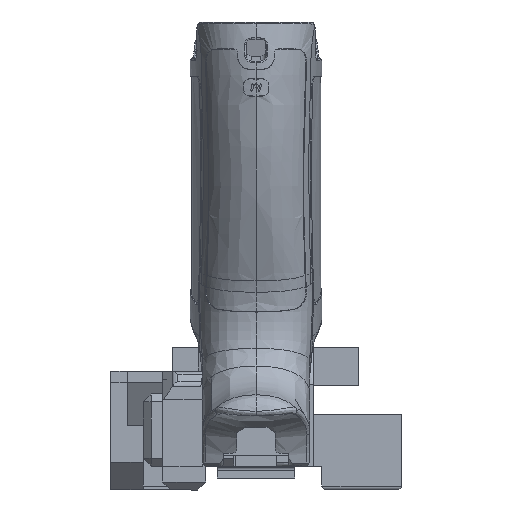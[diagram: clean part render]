
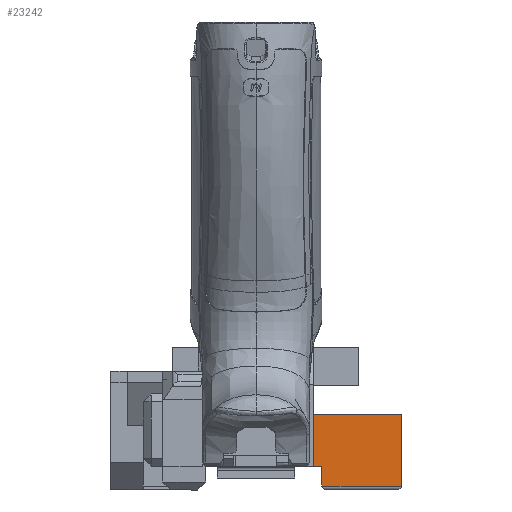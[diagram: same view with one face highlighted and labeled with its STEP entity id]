
A CAD part, left-side view. The second image highlights one B-rep face of the part: STEP entity #23242.
In plain terms, the highlighted planar face has unit normal (-1, 0, 0).
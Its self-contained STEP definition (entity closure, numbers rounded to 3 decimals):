
#552=CIRCLE('',#24701,3.);
#1266=PLANE('',#24794);
#2491=FACE_OUTER_BOUND('',#3825,.T.);
#3825=EDGE_LOOP('',(#18093,#18094,#18095,#18096,#18097,#18098,#18099));
#6152=LINE('',#62624,#8040);
#6186=LINE('',#62721,#8074);
#6187=LINE('',#62723,#8075);
#6188=LINE('',#62725,#8076);
#6189=LINE('',#62726,#8077);
#6190=LINE('',#62727,#8078);
#8040=VECTOR('',#27793,10.);
#8074=VECTOR('',#27853,10.);
#8075=VECTOR('',#27854,10.);
#8076=VECTOR('',#27855,10.);
#8077=VECTOR('',#27856,10.);
#8078=VECTOR('',#27857,10.);
#10216=VERTEX_POINT('',#59979);
#10222=VERTEX_POINT('',#60356);
#10321=VERTEX_POINT('',#62622);
#10356=VERTEX_POINT('',#62719);
#10357=VERTEX_POINT('',#62720);
#10358=VERTEX_POINT('',#62722);
#10359=VERTEX_POINT('',#62724);
#12967=EDGE_CURVE('',#10216,#10222,#552,.T.);
#13136=EDGE_CURVE('',#10216,#10321,#6152,.T.);
#13178=EDGE_CURVE('',#10356,#10357,#6186,.T.);
#13179=EDGE_CURVE('',#10358,#10356,#6187,.T.);
#13180=EDGE_CURVE('',#10359,#10358,#6188,.T.);
#13181=EDGE_CURVE('',#10222,#10359,#6189,.T.);
#13182=EDGE_CURVE('',#10321,#10357,#6190,.T.);
#18093=ORIENTED_EDGE('',*,*,#13178,.F.);
#18094=ORIENTED_EDGE('',*,*,#13179,.F.);
#18095=ORIENTED_EDGE('',*,*,#13180,.F.);
#18096=ORIENTED_EDGE('',*,*,#13181,.F.);
#18097=ORIENTED_EDGE('',*,*,#12967,.F.);
#18098=ORIENTED_EDGE('',*,*,#13136,.T.);
#18099=ORIENTED_EDGE('',*,*,#13182,.T.);
#23242=ADVANCED_FACE('',(#2491),#1266,.T.);
#24701=AXIS2_PLACEMENT_3D('',#60357,#27545,#27546);
#24794=AXIS2_PLACEMENT_3D('',#62718,#27851,#27852);
#27545=DIRECTION('center_axis',(-1.,0.,
0.));
#27546=DIRECTION('ref_axis',(0.,0.,-1.));
#27793=DIRECTION('',(0.,0.,-1.));
#27851=DIRECTION('center_axis',(-1.,0.,
0.));
#27852=DIRECTION('ref_axis',(0.,1.,0.));
#27853=DIRECTION('',(0.,0.,1.));
#27854=DIRECTION('',(0.,1.,0.));
#27855=DIRECTION('',(0.,0.,-1.));
#27856=DIRECTION('',(0.,-1.,0.));
#27857=DIRECTION('',(0.,1.,0.));
#59979=CARTESIAN_POINT('',(-6.591,44.245,-11.946));
#60356=CARTESIAN_POINT('',(-6.591,42.095,-12.854));
#60357=CARTESIAN_POINT('Origin',(-6.591,42.095,-9.854));
#62622=CARTESIAN_POINT('',(-6.591,44.245,-15.026));
#62624=CARTESIAN_POINT('',(-6.591,44.245,-12.854));
#62718=CARTESIAN_POINT('Origin',(-6.591,31.353,-12.854));
#62719=CARTESIAN_POINT('',(-6.591,49.245,-35.025));
#62720=CARTESIAN_POINT('',(-6.591,49.245,-15.026));
#62721=CARTESIAN_POINT('',(-6.591,49.245,-17.897));
#62722=CARTESIAN_POINT('',(-6.591,31.353,-35.025));
#62723=CARTESIAN_POINT('',(-6.591,34.576,-35.025));
#62724=CARTESIAN_POINT('',(-6.591,31.353,-12.854));
#62725=CARTESIAN_POINT('',(-6.591,31.353,-12.854));
#62726=CARTESIAN_POINT('',(-6.591,38.549,-12.854));
#62727=CARTESIAN_POINT('',(-6.591,44.245,-15.026));
